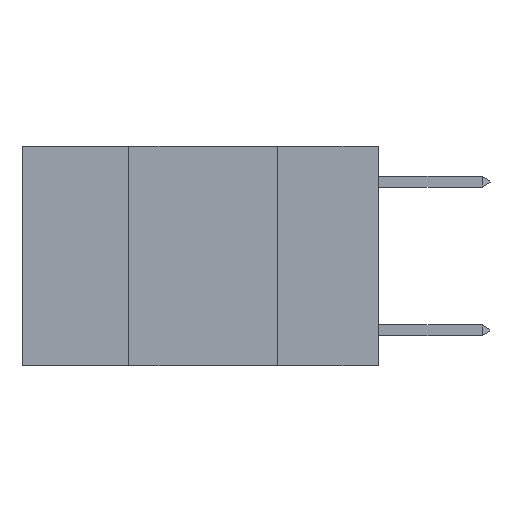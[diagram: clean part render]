
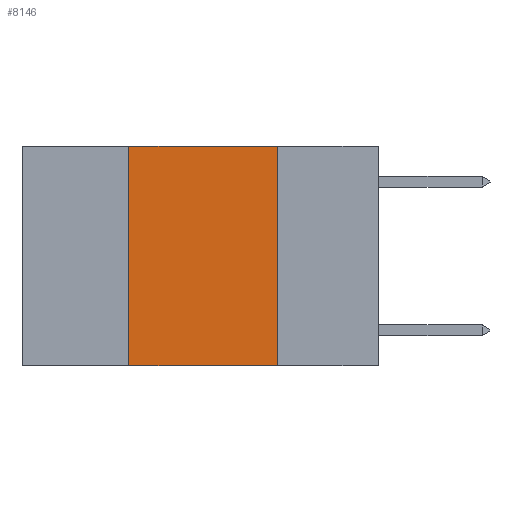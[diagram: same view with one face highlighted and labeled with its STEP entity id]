
A CAD part, left-side view. The second image highlights one B-rep face of the part: STEP entity #8146.
In plain terms, the highlighted planar face has unit normal (-1, 0, 0).
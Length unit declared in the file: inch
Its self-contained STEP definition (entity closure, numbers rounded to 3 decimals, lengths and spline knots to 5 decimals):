
#509 = LINE ( 'NONE', #4475, #5059 ) ;
#532 = LINE ( 'NONE', #722, #1910 ) ;
#649 = VERTEX_POINT ( 'NONE', #5216 ) ;
#722 = CARTESIAN_POINT ( 'NONE',  ( 0., 0.42, 0. ) ) ;
#926 = EDGE_CURVE ( 'NONE', #6973, #5022, #4495, .T. ) ;
#1215 = CARTESIAN_POINT ( 'NONE',  ( 0., 0.17, 0. ) ) ;
#1462 = DIRECTION ( 'NONE',  ( 1., 0., 0. ) ) ;
#1483 = ORIENTED_EDGE ( 'NONE', *, *, #4534, .F. ) ;
#1898 = VECTOR ( 'NONE', #3855, 39.37008 ) ;
#1910 = VECTOR ( 'NONE', #5853, 39.37008 ) ;
#2242 = VECTOR ( 'NONE', #7095, 39.37008 ) ;
#2485 = CARTESIAN_POINT ( 'NONE',  ( 0., 0.6, 0. ) ) ;
#2904 = EDGE_CURVE ( 'NONE', #649, #3533, #509, .T. ) ;
#3533 = VERTEX_POINT ( 'NONE', #7218 ) ;
#3855 = DIRECTION ( 'NONE',  ( 0., 0., -1. ) ) ;
#4125 = FACE_OUTER_BOUND ( 'NONE', #7999, .T. ) ;
#4475 = CARTESIAN_POINT ( 'NONE',  ( 0., 0.6, -0.37 ) ) ;
#4495 = LINE ( 'NONE', #2485, #2242 ) ;
#4508 = DIRECTION ( 'NONE',  ( 0., -1., 0. ) ) ;
#4534 = EDGE_CURVE ( 'NONE', #5022, #3533, #4611, .T. ) ;
#4611 = LINE ( 'NONE', #1215, #1898 ) ;
#4801 = ORIENTED_EDGE ( 'NONE', *, *, #926, .F. ) ;
#4961 = CARTESIAN_POINT ( 'NONE',  ( 0., 0.17, 0. ) ) ;
#5022 = VERTEX_POINT ( 'NONE', #4961 ) ;
#5059 = VECTOR ( 'NONE', #4508, 39.37008 ) ;
#5216 = CARTESIAN_POINT ( 'NONE',  ( 0., 0.42, -0.37 ) ) ;
#5393 = DIRECTION ( 'NONE',  ( 0., 0., -1. ) ) ;
#5443 = PLANE ( 'NONE',  #7476 ) ;
#5733 = EDGE_CURVE ( 'NONE', #649, #6973, #532, .T. ) ;
#5853 = DIRECTION ( 'NONE',  ( 0., 0., 1. ) ) ;
#6103 = CARTESIAN_POINT ( 'NONE',  ( 0., 0.6, 0. ) ) ;
#6596 = ORIENTED_EDGE ( 'NONE', *, *, #5733, .F. ) ;
#6968 = ORIENTED_EDGE ( 'NONE', *, *, #2904, .T. ) ;
#6973 = VERTEX_POINT ( 'NONE', #7520 ) ;
#7095 = DIRECTION ( 'NONE',  ( 0., -1., 0. ) ) ;
#7218 = CARTESIAN_POINT ( 'NONE',  ( 0., 0.17, -0.37 ) ) ;
#7476 = AXIS2_PLACEMENT_3D ( 'NONE', #6103, #1462, #5393 ) ;
#7520 = CARTESIAN_POINT ( 'NONE',  ( 0., 0.42, 0. ) ) ;
#7999 = EDGE_LOOP ( 'NONE', ( #1483, #4801, #6596, #6968 ) ) ;
#8146 = ADVANCED_FACE ( 'NONE', ( #4125 ), #5443, .F. ) ;
